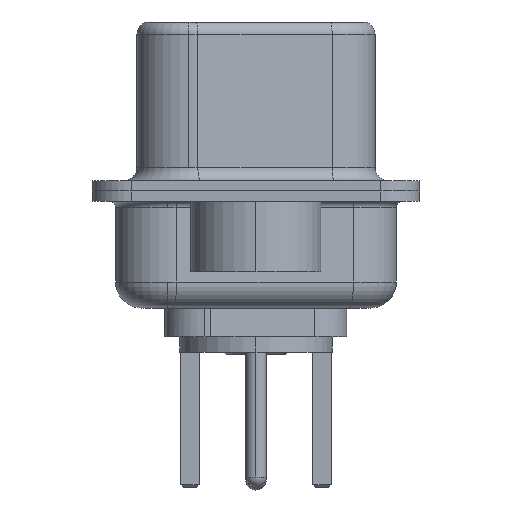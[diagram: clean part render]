
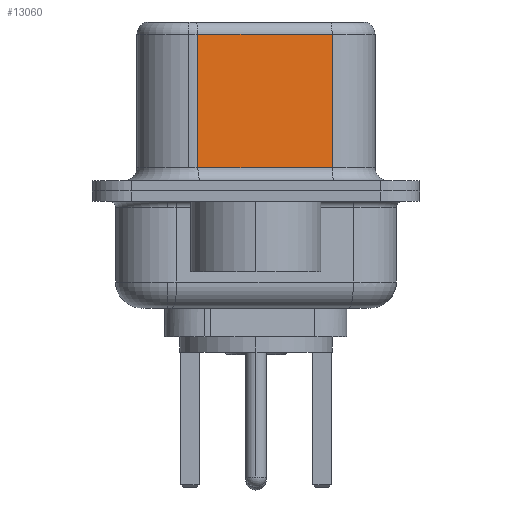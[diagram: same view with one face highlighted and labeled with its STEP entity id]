
A CAD part, left-side view. The second image highlights one B-rep face of the part: STEP entity #13060.
In plain terms, the highlighted planar face has unit normal (-0.985, -0.174, 0).
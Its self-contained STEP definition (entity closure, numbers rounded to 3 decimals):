
#542 = VECTOR ( 'NONE', #15915, 1000. ) ;
#861 = EDGE_CURVE ( 'NONE', #8308, #5477, #5851, .T. ) ;
#1384 = EDGE_LOOP ( 'NONE', ( #1919, #8096, #17810, #17871 ) ) ;
#1500 = CARTESIAN_POINT ( 'NONE',  ( 4.565, -2.927, 6.02 ) ) ;
#1919 = ORIENTED_EDGE ( 'NONE', *, *, #12332, .F. ) ;
#3430 = DIRECTION ( 'NONE',  ( 0., 0., -1. ) ) ;
#3785 = VERTEX_POINT ( 'NONE', #11964 ) ;
#3816 = CARTESIAN_POINT ( 'NONE',  ( 4.565, -2.927, 0.9 ) ) ;
#4446 = CARTESIAN_POINT ( 'NONE',  ( 3.655, 2.233, 6.02 ) ) ;
#5477 = VERTEX_POINT ( 'NONE', #4446 ) ;
#5851 = LINE ( 'NONE', #1500, #14577 ) ;
#6612 = EDGE_CURVE ( 'NONE', #21238, #3785, #13781, .T. ) ;
#6959 = DIRECTION ( 'NONE',  ( 0.985, 0.174, 0. ) ) ;
#7316 = LINE ( 'NONE', #13777, #11966 ) ;
#8096 = ORIENTED_EDGE ( 'NONE', *, *, #861, .T. ) ;
#8308 = VERTEX_POINT ( 'NONE', #11587 ) ;
#8905 = FACE_OUTER_BOUND ( 'NONE', #1384, .T. ) ;
#11468 = VECTOR ( 'NONE', #12627, 1000. ) ;
#11587 = CARTESIAN_POINT ( 'NONE',  ( 4.565, -2.927, 6.02 ) ) ;
#11964 = CARTESIAN_POINT ( 'NONE',  ( 4.565, -2.927, 0.9 ) ) ;
#11966 = VECTOR ( 'NONE', #3430, 1000. ) ;
#12177 = CARTESIAN_POINT ( 'NONE',  ( 4.565, -2.927, 6.52 ) ) ;
#12332 = EDGE_CURVE ( 'NONE', #8308, #3785, #7316, .T. ) ;
#12627 = DIRECTION ( 'NONE',  ( 0., 0., -1. ) ) ;
#13060 = ADVANCED_FACE ( 'NONE', ( #8905 ), #17344, .F. ) ;
#13777 = CARTESIAN_POINT ( 'NONE',  ( 4.565, -2.927, 6.52 ) ) ;
#13781 = LINE ( 'NONE', #3816, #542 ) ;
#14577 = VECTOR ( 'NONE', #15540, 1000. ) ;
#14786 = CARTESIAN_POINT ( 'NONE',  ( 3.655, 2.233, 0.9 ) ) ;
#15540 = DIRECTION ( 'NONE',  ( -0.174, 0.985, 0. ) ) ;
#15555 = AXIS2_PLACEMENT_3D ( 'NONE', #12177, #6959, #18995 ) ;
#15915 = DIRECTION ( 'NONE',  ( 0.174, -0.985, 0. ) ) ;
#17344 = PLANE ( 'NONE',  #15555 ) ;
#17810 = ORIENTED_EDGE ( 'NONE', *, *, #19638, .T. ) ;
#17871 = ORIENTED_EDGE ( 'NONE', *, *, #6612, .T. ) ;
#18995 = DIRECTION ( 'NONE',  ( -0.174, 0.985, 0. ) ) ;
#19638 = EDGE_CURVE ( 'NONE', #5477, #21238, #21080, .T. ) ;
#21080 = LINE ( 'NONE', #21104, #11468 ) ;
#21104 = CARTESIAN_POINT ( 'NONE',  ( 3.655, 2.233, 6.52 ) ) ;
#21238 = VERTEX_POINT ( 'NONE', #14786 ) ;
